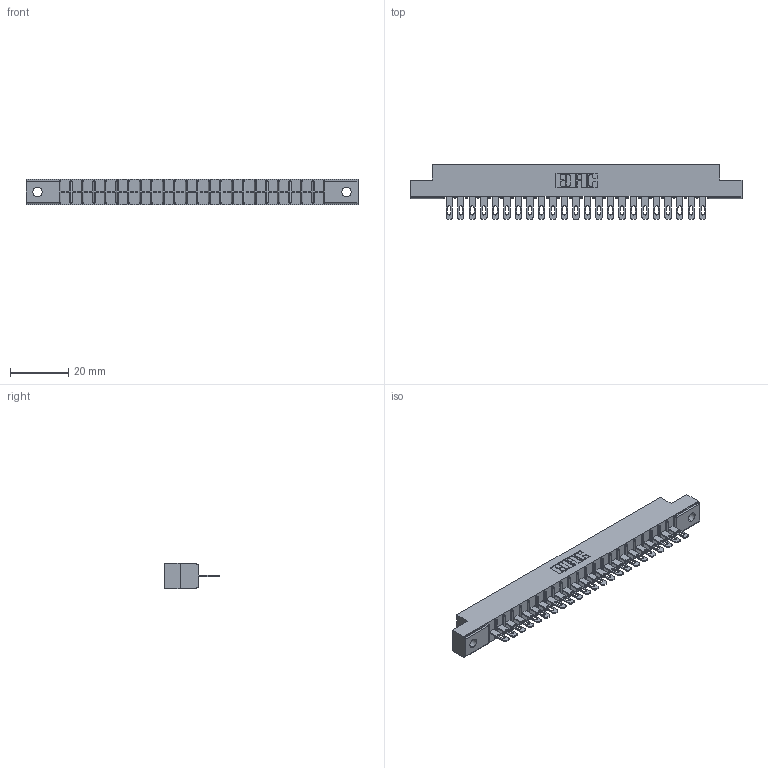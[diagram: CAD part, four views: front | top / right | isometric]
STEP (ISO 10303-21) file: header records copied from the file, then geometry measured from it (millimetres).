
FILE_DESCRIPTION (( 'STEP AP203' ), '1' );
FILE_NAME ('356-023-400-102.STEP', '2020-09-23T15:40:17', ( '' ), ( '' ), 'SwSTEP 2.0', 'SolidWorks 2020', '' );
FILE_SCHEMA (( 'CONFIG_CONTROL_DESIGN' ));
Length unit declared in the file: inch
Products named in the file (3): 306 Part_.128 Dia; 356-023-400-102; 306-290-001_100
Assembly tree (24 placements, depth 2):
  356-023-400-102
    306 Part_.128 Dia
    306-290-001_100  x23
Bounding box: 114.15 x 18.87 x 8.71 mm (x, y, z)
Volume: 7844.5 mm3; surface area: 11743.6 mm2
Topology: 24 solids, 24 shells, 1864 faces, 5261 edges, 3382 vertices
Faces by surface type: plane 1218, cylinder 554, sphere 92
Entity records: 24076 total; most frequent: CARTESIAN_POINT 4040, ORIENTED_EDGE 4002, DIRECTION 3987, EDGE_CURVE 2001, VECTOR 1553, LINE 1553, VERTEX_POINT 1270, AXIS2_PLACEMENT_3D 1217
